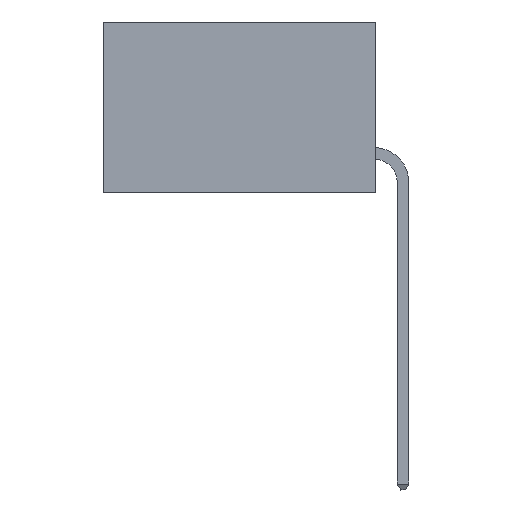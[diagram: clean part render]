
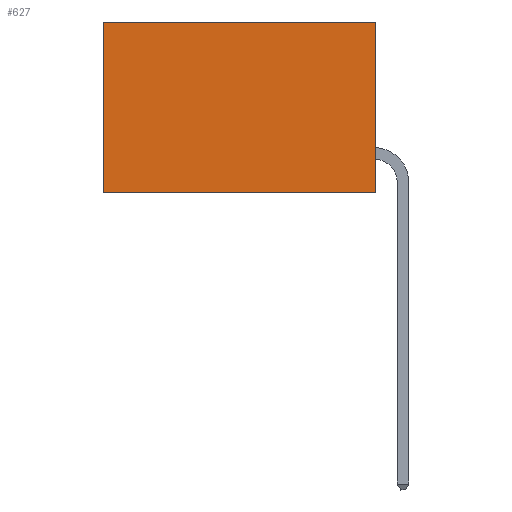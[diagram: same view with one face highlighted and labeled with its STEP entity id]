
A CAD part, left-side view. The second image highlights one B-rep face of the part: STEP entity #627.
In plain terms, the highlighted planar face has unit normal (-1, 0, 0).
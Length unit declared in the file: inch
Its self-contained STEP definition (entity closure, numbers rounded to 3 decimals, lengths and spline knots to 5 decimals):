
#391 = VERTEX_POINT ( 'NONE', #10416 ) ;
#393 = CARTESIAN_POINT ( 'NONE',  ( 0.277, 0., 0. ) ) ;
#627 = ADVANCED_FACE ( 'NONE', ( #2289 ), #5626, .F. ) ;
#1085 = DIRECTION ( 'NONE',  ( 0., 0., -1. ) ) ;
#1546 = LINE ( 'NONE', #8158, #10202 ) ;
#2080 = CARTESIAN_POINT ( 'NONE',  ( 0.277, 0., -0.37 ) ) ;
#2198 = LINE ( 'NONE', #14024, #7910 ) ;
#2289 = FACE_OUTER_BOUND ( 'NONE', #9989, .T. ) ;
#2459 = CARTESIAN_POINT ( 'NONE',  ( 0.277, 0., -0.37 ) ) ;
#2676 = LINE ( 'NONE', #2459, #13669 ) ;
#3504 = VERTEX_POINT ( 'NONE', #10240 ) ;
#4775 = CARTESIAN_POINT ( 'NONE',  ( 0.277, 0.59, 0. ) ) ;
#5626 = PLANE ( 'NONE',  #5754 ) ;
#5754 = AXIS2_PLACEMENT_3D ( 'NONE', #2080, #11463, #11494 ) ;
#5801 = DIRECTION ( 'NONE',  ( 0., 0., -1. ) ) ;
#5999 = ORIENTED_EDGE ( 'NONE', *, *, #12415, .T. ) ;
#6222 = ORIENTED_EDGE ( 'NONE', *, *, #11384, .F. ) ;
#6318 = ORIENTED_EDGE ( 'NONE', *, *, #8371, .F. ) ;
#6409 = ORIENTED_EDGE ( 'NONE', *, *, #6512, .T. ) ;
#6512 = EDGE_CURVE ( 'NONE', #8343, #391, #12347, .T. ) ;
#7847 = VERTEX_POINT ( 'NONE', #393 ) ;
#7910 = VECTOR ( 'NONE', #1085, 39.37008 ) ;
#8158 = CARTESIAN_POINT ( 'NONE',  ( 0.277, 0., 0. ) ) ;
#8343 = VERTEX_POINT ( 'NONE', #4775 ) ;
#8371 = EDGE_CURVE ( 'NONE', #3504, #391, #2676, .T. ) ;
#9228 = DIRECTION ( 'NONE',  ( 0., 1., 0. ) ) ;
#9273 = DIRECTION ( 'NONE',  ( 0., 1., 0. ) ) ;
#9391 = VECTOR ( 'NONE', #5801, 39.37008 ) ;
#9989 = EDGE_LOOP ( 'NONE', ( #6409, #6318, #6222, #5999 ) ) ;
#10202 = VECTOR ( 'NONE', #9273, 39.37008 ) ;
#10240 = CARTESIAN_POINT ( 'NONE',  ( 0.277, 0., -0.37 ) ) ;
#10416 = CARTESIAN_POINT ( 'NONE',  ( 0.277, 0.59, -0.37 ) ) ;
#11159 = CARTESIAN_POINT ( 'NONE',  ( 0.277, 0.59, -0.37 ) ) ;
#11384 = EDGE_CURVE ( 'NONE', #7847, #3504, #2198, .T. ) ;
#11463 = DIRECTION ( 'NONE',  ( 1., 0., 0. ) ) ;
#11494 = DIRECTION ( 'NONE',  ( 0., 0., -1. ) ) ;
#12347 = LINE ( 'NONE', #11159, #9391 ) ;
#12415 = EDGE_CURVE ( 'NONE', #7847, #8343, #1546, .T. ) ;
#13669 = VECTOR ( 'NONE', #9228, 39.37008 ) ;
#14024 = CARTESIAN_POINT ( 'NONE',  ( 0.277, 0., -0.37 ) ) ;
